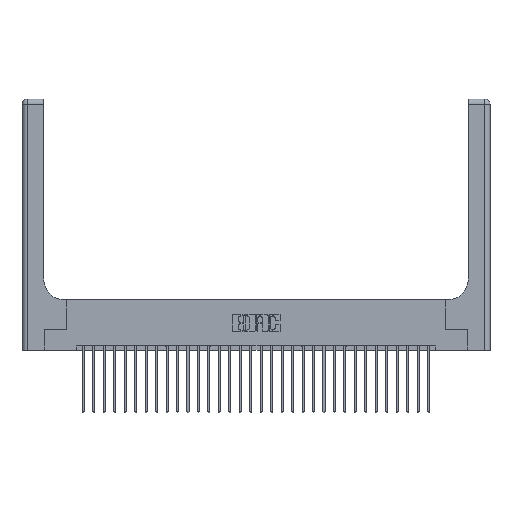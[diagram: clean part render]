
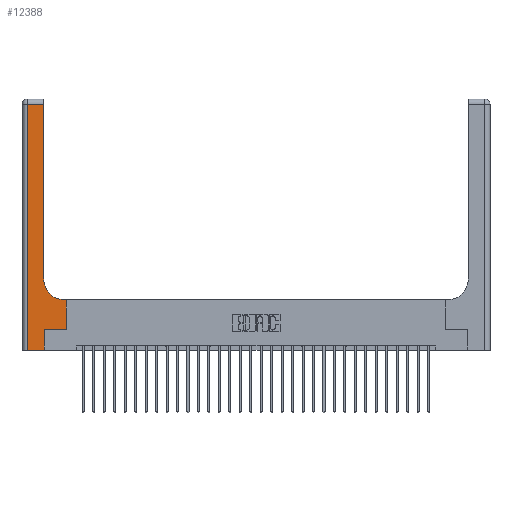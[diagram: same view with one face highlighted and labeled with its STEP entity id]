
A CAD part, top view. The second image highlights one B-rep face of the part: STEP entity #12388.
In plain terms, the highlighted planar face has unit normal (0, 0, 1).
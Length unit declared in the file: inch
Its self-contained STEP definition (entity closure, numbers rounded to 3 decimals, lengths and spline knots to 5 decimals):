
#458 = LINE ( 'NONE', #2359, #2042 ) ;
#1520 = VERTEX_POINT ( 'NONE', #11332 ) ;
#2006 = ORIENTED_EDGE ( 'NONE', *, *, #15967, .T. ) ;
#2042 = VECTOR ( 'NONE', #7345, 39.37008 ) ;
#2196 = VECTOR ( 'NONE', #19459, 39.37008 ) ;
#2359 = CARTESIAN_POINT ( 'NONE',  ( 0.265, 0.25, 0.37 ) ) ;
#2438 = LINE ( 'NONE', #15885, #20902 ) ;
#2478 = ORIENTED_EDGE ( 'NONE', *, *, #4819, .T. ) ;
#2830 = DIRECTION ( 'NONE',  ( -1., 0., 0. ) ) ;
#3311 = VERTEX_POINT ( 'NONE', #7781 ) ;
#3685 = VECTOR ( 'NONE', #15008, 39.37008 ) ;
#3761 = CIRCLE ( 'NONE', #4227, 0.25 ) ;
#3919 = VECTOR ( 'NONE', #11375, 39.37008 ) ;
#4187 = DIRECTION ( 'NONE',  ( -1., 0., 0. ) ) ;
#4227 = AXIS2_PLACEMENT_3D ( 'NONE', #7947, #16846, #12620 ) ;
#4394 = EDGE_CURVE ( 'NONE', #1520, #13361, #9699, .T. ) ;
#4420 = VECTOR ( 'NONE', #2830, 39.37008 ) ;
#4546 = CARTESIAN_POINT ( 'NONE',  ( 0.06, 3., 0.37 ) ) ;
#4691 = CARTESIAN_POINT ( 'NONE',  ( 0.265, 0.25, 0.37 ) ) ;
#4819 = EDGE_CURVE ( 'NONE', #4963, #7292, #458, .T. ) ;
#4963 = VERTEX_POINT ( 'NONE', #4691 ) ;
#5075 = LINE ( 'NONE', #9166, #3919 ) ;
#5484 = VERTEX_POINT ( 'NONE', #17461 ) ;
#5829 = VECTOR ( 'NONE', #16212, 39.37008 ) ;
#5855 = ORIENTED_EDGE ( 'NONE', *, *, #18689, .T. ) ;
#6494 = CARTESIAN_POINT ( 'NONE',  ( 0.528, 0.6, 0.37 ) ) ;
#6665 = CARTESIAN_POINT ( 'NONE',  ( 0.265, 0., 0.37 ) ) ;
#7011 = EDGE_CURVE ( 'NONE', #5484, #3311, #5075, .T. ) ;
#7039 = ORIENTED_EDGE ( 'NONE', *, *, #22315, .T. ) ;
#7292 = VERTEX_POINT ( 'NONE', #27764 ) ;
#7345 = DIRECTION ( 'NONE',  ( 1., 0., 0. ) ) ;
#7781 = CARTESIAN_POINT ( 'NONE',  ( 0.265, 0., 0.37 ) ) ;
#7947 = CARTESIAN_POINT ( 'NONE',  ( 0.51, 0.85, 0.37 ) ) ;
#7992 = CARTESIAN_POINT ( 'NONE',  ( 0., 3., 0.37 ) ) ;
#8962 = DIRECTION ( 'NONE',  ( 0., 1., 0. ) ) ;
#9166 = CARTESIAN_POINT ( 'NONE',  ( 0., 0., 0.37 ) ) ;
#9699 = LINE ( 'NONE', #25217, #4420 ) ;
#10482 = VERTEX_POINT ( 'NONE', #6494 ) ;
#10566 = CARTESIAN_POINT ( 'NONE',  ( 0.26, 0.6, 0.37 ) ) ;
#11136 = CARTESIAN_POINT ( 'NONE',  ( 0.06, 2.94, 0.37 ) ) ;
#11332 = CARTESIAN_POINT ( 'NONE',  ( 0.26, 2.94, 0.37 ) ) ;
#11375 = DIRECTION ( 'NONE',  ( 1., 0., 0. ) ) ;
#11571 = LINE ( 'NONE', #4546, #5829 ) ;
#12152 = EDGE_LOOP ( 'NONE', ( #5855, #18174, #20711, #19255, #2006, #2478, #26675, #27630, #7039 ) ) ;
#12388 = ADVANCED_FACE ( 'NONE', ( #19665 ), #15149, .F. ) ;
#12620 = DIRECTION ( 'NONE',  ( 1., 0., 0. ) ) ;
#13361 = VERTEX_POINT ( 'NONE', #11136 ) ;
#15008 = DIRECTION ( 'NONE',  ( 0., 1., 0. ) ) ;
#15149 = PLANE ( 'NONE',  #25129 ) ;
#15706 = LINE ( 'NONE', #6665, #15730 ) ;
#15721 = EDGE_CURVE ( 'NONE', #10482, #20464, #28294, .T. ) ;
#15730 = VECTOR ( 'NONE', #8962, 39.37008 ) ;
#15885 = CARTESIAN_POINT ( 'NONE',  ( 0.26, 3., 0.37 ) ) ;
#15967 = EDGE_CURVE ( 'NONE', #3311, #4963, #15706, .T. ) ;
#16212 = DIRECTION ( 'NONE',  ( 0., -1., 0. ) ) ;
#16846 = DIRECTION ( 'NONE',  ( 0., 0., -1. ) ) ;
#16873 = CARTESIAN_POINT ( 'NONE',  ( 0.51, 0.6, 0.37 ) ) ;
#17461 = CARTESIAN_POINT ( 'NONE',  ( 0.06, 0., 0.37 ) ) ;
#18174 = ORIENTED_EDGE ( 'NONE', *, *, #4394, .T. ) ;
#18529 = VERTEX_POINT ( 'NONE', #24546 ) ;
#18689 = EDGE_CURVE ( 'NONE', #18529, #1520, #2438, .T. ) ;
#19255 = ORIENTED_EDGE ( 'NONE', *, *, #7011, .T. ) ;
#19459 = DIRECTION ( 'NONE',  ( -1., 0., 0. ) ) ;
#19665 = FACE_OUTER_BOUND ( 'NONE', #12152, .T. ) ;
#20053 = EDGE_CURVE ( 'NONE', #7292, #10482, #26150, .T. ) ;
#20263 = DIRECTION ( 'NONE',  ( 0., 1., 0. ) ) ;
#20464 = VERTEX_POINT ( 'NONE', #16873 ) ;
#20711 = ORIENTED_EDGE ( 'NONE', *, *, #25477, .T. ) ;
#20902 = VECTOR ( 'NONE', #20263, 39.37008 ) ;
#21569 = CARTESIAN_POINT ( 'NONE',  ( 0.528, 0.25, 0.37 ) ) ;
#22315 = EDGE_CURVE ( 'NONE', #20464, #18529, #3761, .T. ) ;
#24546 = CARTESIAN_POINT ( 'NONE',  ( 0.26, 0.85, 0.37 ) ) ;
#25129 = AXIS2_PLACEMENT_3D ( 'NONE', #7992, #28357, #4187 ) ;
#25217 = CARTESIAN_POINT ( 'NONE',  ( 0., 2.94, 0.37 ) ) ;
#25477 = EDGE_CURVE ( 'NONE', #13361, #5484, #11571, .T. ) ;
#26150 = LINE ( 'NONE', #21569, #3685 ) ;
#26675 = ORIENTED_EDGE ( 'NONE', *, *, #20053, .T. ) ;
#27630 = ORIENTED_EDGE ( 'NONE', *, *, #15721, .T. ) ;
#27764 = CARTESIAN_POINT ( 'NONE',  ( 0.528, 0.25, 0.37 ) ) ;
#28294 = LINE ( 'NONE', #10566, #2196 ) ;
#28357 = DIRECTION ( 'NONE',  ( 0., 0., -1. ) ) ;
